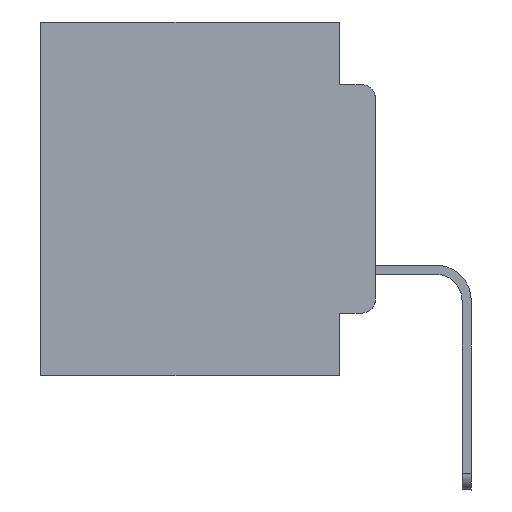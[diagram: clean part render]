
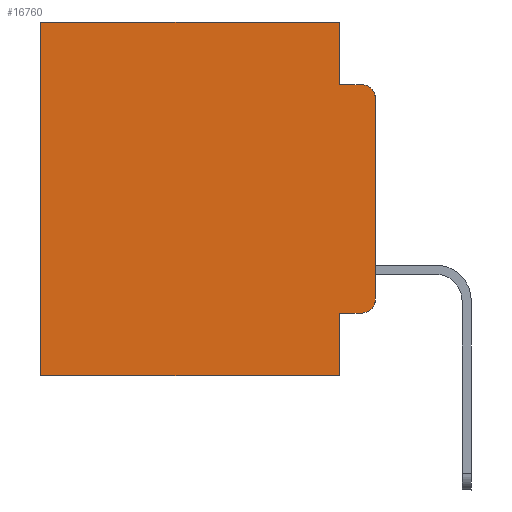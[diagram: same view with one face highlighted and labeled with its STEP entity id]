
A CAD part, left-side view. The second image highlights one B-rep face of the part: STEP entity #16760.
In plain terms, the highlighted planar face has unit normal (-1, 0, 0).
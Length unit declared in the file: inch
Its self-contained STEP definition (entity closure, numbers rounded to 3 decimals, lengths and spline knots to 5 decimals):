
#807 = CARTESIAN_POINT ( 'NONE',  ( 0.298, 0.051, 0. ) ) ;
#1221 = EDGE_LOOP ( 'NONE', ( #24666, #5378, #22235, #27797, #13594, #25437, #21397, #3587, #4384, #19281 ) ) ;
#1387 = VECTOR ( 'NONE', #25068, 39.37008 ) ;
#1640 = EDGE_CURVE ( 'NONE', #11549, #9151, #22771, .T. ) ;
#1707 = LINE ( 'NONE', #9291, #14077 ) ;
#1776 = DIRECTION ( 'NONE',  ( 0., 0., -1. ) ) ;
#1997 = CARTESIAN_POINT ( 'NONE',  ( 0.298, 0.473, 0. ) ) ;
#2228 = CARTESIAN_POINT ( 'NONE',  ( 0.298, 0.051, -0.5 ) ) ;
#2327 = CARTESIAN_POINT ( 'NONE',  ( 0.298, 0.02, -0.1085 ) ) ;
#2416 = FACE_OUTER_BOUND ( 'NONE', #1221, .T. ) ;
#2926 = CIRCLE ( 'NONE', #11961, 0.02 ) ;
#3301 = VERTEX_POINT ( 'NONE', #20771 ) ;
#3351 = CARTESIAN_POINT ( 'NONE',  ( 0.298, 0., 0. ) ) ;
#3392 = VERTEX_POINT ( 'NONE', #13992 ) ;
#3587 = ORIENTED_EDGE ( 'NONE', *, *, #17507, .F. ) ;
#3644 = EDGE_CURVE ( 'NONE', #14834, #26318, #17996, .T. ) ;
#4384 = ORIENTED_EDGE ( 'NONE', *, *, #22637, .T. ) ;
#4404 = CARTESIAN_POINT ( 'NONE',  ( 0.298, 0.051, 0. ) ) ;
#4593 = VECTOR ( 'NONE', #20148, 39.37008 ) ;
#4916 = VECTOR ( 'NONE', #20884, 39.37008 ) ;
#5065 = PLANE ( 'NONE',  #23044 ) ;
#5160 = DIRECTION ( 'NONE',  ( 0., 0., -1. ) ) ;
#5171 = VECTOR ( 'NONE', #20228, 39.37008 ) ;
#5282 = LINE ( 'NONE', #24284, #4593 ) ;
#5378 = ORIENTED_EDGE ( 'NONE', *, *, #25323, .T. ) ;
#5662 = EDGE_CURVE ( 'NONE', #14834, #3301, #1707, .T. ) ;
#7252 = EDGE_CURVE ( 'NONE', #26318, #9925, #16769, .T. ) ;
#7952 = VECTOR ( 'NONE', #22957, 39.37008 ) ;
#7984 = CARTESIAN_POINT ( 'NONE',  ( 0.298, 0., -0.1085 ) ) ;
#8771 = DIRECTION ( 'NONE',  ( -1., 0., 0. ) ) ;
#9151 = VERTEX_POINT ( 'NONE', #19340 ) ;
#9291 = CARTESIAN_POINT ( 'NONE',  ( 0.298, 0.051, 0. ) ) ;
#9356 = CARTESIAN_POINT ( 'NONE',  ( 0.298, 0., 0. ) ) ;
#9925 = VERTEX_POINT ( 'NONE', #24804 ) ;
#10290 = EDGE_CURVE ( 'NONE', #3392, #9151, #14169, .T. ) ;
#10442 = DIRECTION ( 'NONE',  ( 0., 1., 0. ) ) ;
#10481 = CARTESIAN_POINT ( 'NONE',  ( 0.298, 0.473, 0. ) ) ;
#10498 = DIRECTION ( 'NONE',  ( -1., 0., 0. ) ) ;
#10588 = VERTEX_POINT ( 'NONE', #24669 ) ;
#10934 = CARTESIAN_POINT ( 'NONE',  ( 0.298, 0., 0. ) ) ;
#11549 = VERTEX_POINT ( 'NONE', #7984 ) ;
#11961 = AXIS2_PLACEMENT_3D ( 'NONE', #2327, #8771, #19861 ) ;
#12807 = CARTESIAN_POINT ( 'NONE',  ( 0.298, 0.02, -0.3915 ) ) ;
#13058 = LINE ( 'NONE', #807, #1387 ) ;
#13457 = CARTESIAN_POINT ( 'NONE',  ( 0.298, 0.051, -0.4115 ) ) ;
#13594 = ORIENTED_EDGE ( 'NONE', *, *, #3644, .T. ) ;
#13992 = CARTESIAN_POINT ( 'NONE',  ( 0.298, 0.02, -0.4115 ) ) ;
#14077 = VECTOR ( 'NONE', #17371, 39.37008 ) ;
#14158 = EDGE_CURVE ( 'NONE', #22509, #9925, #27765, .T. ) ;
#14169 = CIRCLE ( 'NONE', #16664, 0.02 ) ;
#14226 = CARTESIAN_POINT ( 'NONE',  ( 0.298, 0.051, -0.4115 ) ) ;
#14834 = VERTEX_POINT ( 'NONE', #4404 ) ;
#15492 = EDGE_CURVE ( 'NONE', #3301, #10588, #5282, .T. ) ;
#15656 = VERTEX_POINT ( 'NONE', #14226 ) ;
#16482 = LINE ( 'NONE', #13457, #5171 ) ;
#16664 = AXIS2_PLACEMENT_3D ( 'NONE', #12807, #10498, #1776 ) ;
#16760 = ADVANCED_FACE ( 'NONE', ( #2416 ), #5065, .F. ) ;
#16769 = LINE ( 'NONE', #1997, #17808 ) ;
#17371 = DIRECTION ( 'NONE',  ( 0., 0., -1. ) ) ;
#17392 = DIRECTION ( 'NONE',  ( 0., 0., -1. ) ) ;
#17435 = VECTOR ( 'NONE', #10442, 39.37008 ) ;
#17507 = EDGE_CURVE ( 'NONE', #15656, #22509, #13058, .T. ) ;
#17808 = VECTOR ( 'NONE', #17392, 39.37008 ) ;
#17996 = LINE ( 'NONE', #10934, #4916 ) ;
#18235 = DIRECTION ( 'NONE',  ( 1., 0., 0. ) ) ;
#19281 = ORIENTED_EDGE ( 'NONE', *, *, #10290, .T. ) ;
#19340 = CARTESIAN_POINT ( 'NONE',  ( 0.298, 0., -0.3915 ) ) ;
#19861 = DIRECTION ( 'NONE',  ( 0., 0., -1. ) ) ;
#20148 = DIRECTION ( 'NONE',  ( 0., -1., 0. ) ) ;
#20228 = DIRECTION ( 'NONE',  ( 0., -1., 0. ) ) ;
#20771 = CARTESIAN_POINT ( 'NONE',  ( 0.298, 0.051, -0.0885 ) ) ;
#20884 = DIRECTION ( 'NONE',  ( 0., 1., 0. ) ) ;
#21397 = ORIENTED_EDGE ( 'NONE', *, *, #14158, .F. ) ;
#21487 = CARTESIAN_POINT ( 'NONE',  ( 0.298, 0., -0.5 ) ) ;
#22235 = ORIENTED_EDGE ( 'NONE', *, *, #15492, .F. ) ;
#22509 = VERTEX_POINT ( 'NONE', #2228 ) ;
#22637 = EDGE_CURVE ( 'NONE', #15656, #3392, #16482, .T. ) ;
#22771 = LINE ( 'NONE', #3351, #7952 ) ;
#22957 = DIRECTION ( 'NONE',  ( 0., 0., -1. ) ) ;
#23044 = AXIS2_PLACEMENT_3D ( 'NONE', #9356, #18235, #5160 ) ;
#24284 = CARTESIAN_POINT ( 'NONE',  ( 0.298, 0.051, -0.0885 ) ) ;
#24666 = ORIENTED_EDGE ( 'NONE', *, *, #1640, .F. ) ;
#24669 = CARTESIAN_POINT ( 'NONE',  ( 0.298, 0.02, -0.0885 ) ) ;
#24804 = CARTESIAN_POINT ( 'NONE',  ( 0.298, 0.473, -0.5 ) ) ;
#25068 = DIRECTION ( 'NONE',  ( 0., 0., -1. ) ) ;
#25323 = EDGE_CURVE ( 'NONE', #11549, #10588, #2926, .T. ) ;
#25437 = ORIENTED_EDGE ( 'NONE', *, *, #7252, .T. ) ;
#26318 = VERTEX_POINT ( 'NONE', #10481 ) ;
#27765 = LINE ( 'NONE', #21487, #17435 ) ;
#27797 = ORIENTED_EDGE ( 'NONE', *, *, #5662, .F. ) ;
